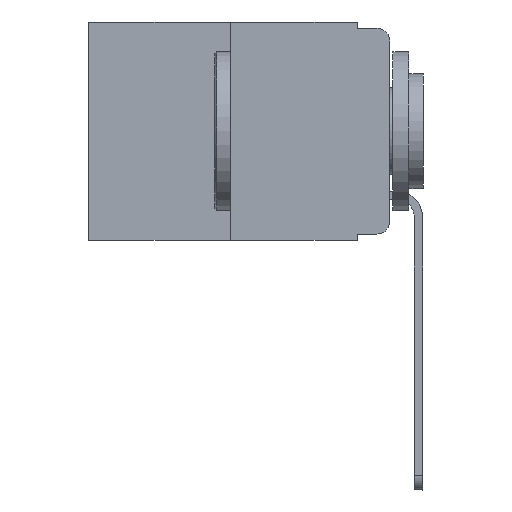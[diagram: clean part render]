
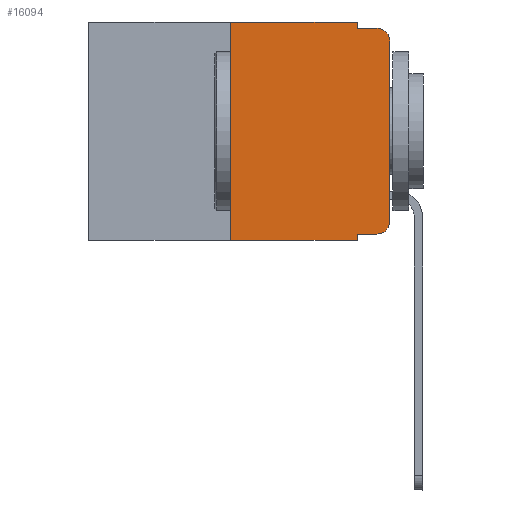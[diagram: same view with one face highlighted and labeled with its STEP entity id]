
A CAD part, left-side view. The second image highlights one B-rep face of the part: STEP entity #16094.
In plain terms, the highlighted planar face has unit normal (-1, 0, 0).
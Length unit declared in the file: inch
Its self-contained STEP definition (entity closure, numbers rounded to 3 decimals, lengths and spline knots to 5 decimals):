
#606 = VERTEX_POINT ( 'NONE', #17546 ) ;
#1022 = AXIS2_PLACEMENT_3D ( 'NONE', #1272, #18196, #16799 ) ;
#1272 = CARTESIAN_POINT ( 'NONE',  ( 0., 0.02, -0.03 ) ) ;
#1390 = LINE ( 'NONE', #6022, #14924 ) ;
#1802 = VERTEX_POINT ( 'NONE', #17180 ) ;
#1907 = CARTESIAN_POINT ( 'NONE',  ( 0., 0.02, -0.333 ) ) ;
#2528 = PLANE ( 'NONE',  #11335 ) ;
#3125 = VECTOR ( 'NONE', #13266, 39.37008 ) ;
#3422 = EDGE_CURVE ( 'NONE', #19262, #15212, #18093, .T. ) ;
#4229 = LINE ( 'NONE', #10380, #3125 ) ;
#4382 = EDGE_CURVE ( 'NONE', #4893, #606, #1390, .T. ) ;
#4778 = ORIENTED_EDGE ( 'NONE', *, *, #3422, .F. ) ;
#4791 = VECTOR ( 'NONE', #4964, 39.37008 ) ;
#4795 = EDGE_CURVE ( 'NONE', #606, #13552, #7028, .T. ) ;
#4893 = VERTEX_POINT ( 'NONE', #9578 ) ;
#4964 = DIRECTION ( 'NONE',  ( 0., 0., -1. ) ) ;
#5261 = DIRECTION ( 'NONE',  ( 0., -1., 0. ) ) ;
#5339 = VECTOR ( 'NONE', #8262, 39.37008 ) ;
#6022 = CARTESIAN_POINT ( 'NONE',  ( 0., 0., 0. ) ) ;
#6030 = AXIS2_PLACEMENT_3D ( 'NONE', #17514, #8501, #7006 ) ;
#6057 = DIRECTION ( 'NONE',  ( 0., -1., 0. ) ) ;
#6079 = CIRCLE ( 'NONE', #6030, 0.02 ) ;
#6239 = CARTESIAN_POINT ( 'NONE',  ( 0., 0.051, -0.01 ) ) ;
#7006 = DIRECTION ( 'NONE',  ( 0., 0., -1. ) ) ;
#7028 = CIRCLE ( 'NONE', #1022, 0.02 ) ;
#7076 = EDGE_CURVE ( 'NONE', #15335, #15588, #7552, .T. ) ;
#7084 = ORIENTED_EDGE ( 'NONE', *, *, #12934, .F. ) ;
#7109 = DIRECTION ( 'NONE',  ( 0., 0., -1. ) ) ;
#7229 = DIRECTION ( 'NONE',  ( 0., 0., 1. ) ) ;
#7286 = VECTOR ( 'NONE', #7109, 39.37008 ) ;
#7552 = LINE ( 'NONE', #12427, #4791 ) ;
#8261 = EDGE_CURVE ( 'NONE', #14227, #4893, #6079, .T. ) ;
#8262 = DIRECTION ( 'NONE',  ( 0., -1., 0. ) ) ;
#8364 = LINE ( 'NONE', #17480, #5339 ) ;
#8474 = CARTESIAN_POINT ( 'NONE',  ( 0., 0.473, 0. ) ) ;
#8501 = DIRECTION ( 'NONE',  ( -1., 0., 0. ) ) ;
#8564 = DIRECTION ( 'NONE',  ( 0., 0., -1. ) ) ;
#9364 = VECTOR ( 'NONE', #6057, 39.37008 ) ;
#9566 = ORIENTED_EDGE ( 'NONE', *, *, #4382, .T. ) ;
#9578 = CARTESIAN_POINT ( 'NONE',  ( 0., 0., -0.313 ) ) ;
#9641 = ORIENTED_EDGE ( 'NONE', *, *, #15534, .T. ) ;
#9682 = VECTOR ( 'NONE', #5261, 39.37008 ) ;
#10089 = CARTESIAN_POINT ( 'NONE',  ( 0., 0.051, 0. ) ) ;
#10380 = CARTESIAN_POINT ( 'NONE',  ( 0., 0.25, 0. ) ) ;
#10438 = VERTEX_POINT ( 'NONE', #17959 ) ;
#10535 = LINE ( 'NONE', #10931, #9364 ) ;
#10931 = CARTESIAN_POINT ( 'NONE',  ( 0., 0.051, -0.01 ) ) ;
#11324 = VECTOR ( 'NONE', #14048, 39.37008 ) ;
#11335 = AXIS2_PLACEMENT_3D ( 'NONE', #8474, #15818, #8564 ) ;
#11985 = EDGE_CURVE ( 'NONE', #19262, #14227, #18603, .T. ) ;
#12242 = CARTESIAN_POINT ( 'NONE',  ( 0., 0.051, -0.333 ) ) ;
#12427 = CARTESIAN_POINT ( 'NONE',  ( 0., 0.051, 0. ) ) ;
#12687 = ORIENTED_EDGE ( 'NONE', *, *, #11985, .T. ) ;
#12818 = LINE ( 'NONE', #18850, #9682 ) ;
#12934 = EDGE_CURVE ( 'NONE', #15588, #13552, #10535, .T. ) ;
#13041 = ORIENTED_EDGE ( 'NONE', *, *, #17415, .F. ) ;
#13125 = EDGE_CURVE ( 'NONE', #10438, #15335, #12818, .T. ) ;
#13266 = DIRECTION ( 'NONE',  ( 0., 0., 1. ) ) ;
#13314 = EDGE_LOOP ( 'NONE', ( #9566, #14241, #7084, #13830, #16091, #13041, #9641, #4778, #12687, #18086 ) ) ;
#13552 = VERTEX_POINT ( 'NONE', #17040 ) ;
#13830 = ORIENTED_EDGE ( 'NONE', *, *, #7076, .F. ) ;
#14048 = DIRECTION ( 'NONE',  ( 0., -1., 0. ) ) ;
#14227 = VERTEX_POINT ( 'NONE', #1907 ) ;
#14241 = ORIENTED_EDGE ( 'NONE', *, *, #4795, .T. ) ;
#14924 = VECTOR ( 'NONE', #7229, 39.37008 ) ;
#15212 = VERTEX_POINT ( 'NONE', #17111 ) ;
#15335 = VERTEX_POINT ( 'NONE', #16224 ) ;
#15434 = CARTESIAN_POINT ( 'NONE',  ( 0., 0.051, -0.333 ) ) ;
#15534 = EDGE_CURVE ( 'NONE', #1802, #15212, #8364, .T. ) ;
#15588 = VERTEX_POINT ( 'NONE', #6239 ) ;
#15818 = DIRECTION ( 'NONE',  ( 1., 0., 0. ) ) ;
#16091 = ORIENTED_EDGE ( 'NONE', *, *, #13125, .F. ) ;
#16094 = ADVANCED_FACE ( 'NONE', ( #17778 ), #2528, .F. ) ;
#16224 = CARTESIAN_POINT ( 'NONE',  ( 0., 0.051, 0. ) ) ;
#16799 = DIRECTION ( 'NONE',  ( 0., 0., -1. ) ) ;
#17040 = CARTESIAN_POINT ( 'NONE',  ( 0., 0.02, -0.01 ) ) ;
#17111 = CARTESIAN_POINT ( 'NONE',  ( 0., 0.051, -0.343 ) ) ;
#17180 = CARTESIAN_POINT ( 'NONE',  ( 0., 0.25, -0.343 ) ) ;
#17415 = EDGE_CURVE ( 'NONE', #1802, #10438, #4229, .T. ) ;
#17480 = CARTESIAN_POINT ( 'NONE',  ( 0., 0.473, -0.343 ) ) ;
#17514 = CARTESIAN_POINT ( 'NONE',  ( 0., 0.02, -0.313 ) ) ;
#17546 = CARTESIAN_POINT ( 'NONE',  ( 0., 0., -0.03 ) ) ;
#17778 = FACE_OUTER_BOUND ( 'NONE', #13314, .T. ) ;
#17959 = CARTESIAN_POINT ( 'NONE',  ( 0., 0.25, 0. ) ) ;
#18086 = ORIENTED_EDGE ( 'NONE', *, *, #8261, .T. ) ;
#18093 = LINE ( 'NONE', #10089, #7286 ) ;
#18196 = DIRECTION ( 'NONE',  ( -1., 0., 0. ) ) ;
#18603 = LINE ( 'NONE', #15434, #11324 ) ;
#18850 = CARTESIAN_POINT ( 'NONE',  ( 0., 0.473, 0. ) ) ;
#19262 = VERTEX_POINT ( 'NONE', #12242 ) ;
